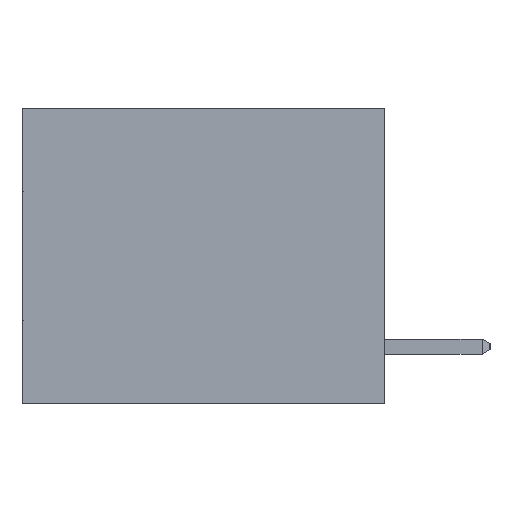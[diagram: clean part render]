
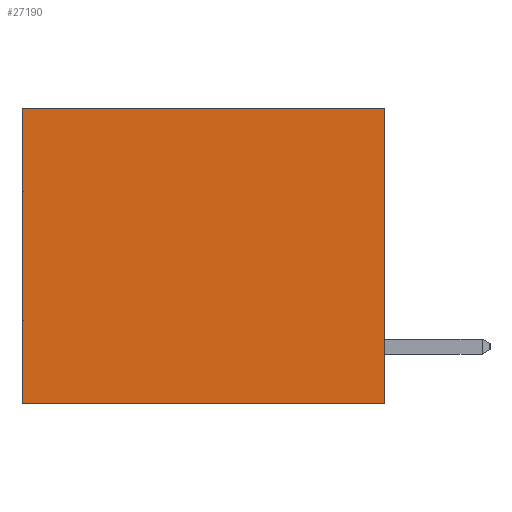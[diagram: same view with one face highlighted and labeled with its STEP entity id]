
A CAD part, left-side view. The second image highlights one B-rep face of the part: STEP entity #27190.
In plain terms, the highlighted planar face has unit normal (-1, 0, 0).
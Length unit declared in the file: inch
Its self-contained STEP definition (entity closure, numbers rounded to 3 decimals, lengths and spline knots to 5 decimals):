
#193 = DIRECTION ( 'NONE',  ( 0., 1., 0. ) ) ;
#298 = CARTESIAN_POINT ( 'NONE',  ( 0.3165, 0., -0.49 ) ) ;
#2090 = EDGE_CURVE ( 'NONE', #5669, #10678, #21121, .T. ) ;
#2999 = CARTESIAN_POINT ( 'NONE',  ( 0.3165, 0.6, -0.49 ) ) ;
#3808 = VECTOR ( 'NONE', #22911, 39.37008 ) ;
#4365 = DIRECTION ( 'NONE',  ( 0., 0., -1. ) ) ;
#4536 = DIRECTION ( 'NONE',  ( 0., 0., -1. ) ) ;
#5238 = ORIENTED_EDGE ( 'NONE', *, *, #6955, .F. ) ;
#5669 = VERTEX_POINT ( 'NONE', #9580 ) ;
#6796 = ORIENTED_EDGE ( 'NONE', *, *, #2090, .T. ) ;
#6955 = EDGE_CURVE ( 'NONE', #12407, #9660, #8573, .T. ) ;
#7861 = CARTESIAN_POINT ( 'NONE',  ( 0.3165, 0., 0. ) ) ;
#8573 = LINE ( 'NONE', #22320, #17529 ) ;
#9580 = CARTESIAN_POINT ( 'NONE',  ( 0.3165, 0.6, 0. ) ) ;
#9660 = VERTEX_POINT ( 'NONE', #25773 ) ;
#10678 = VERTEX_POINT ( 'NONE', #2999 ) ;
#11215 = DIRECTION ( 'NONE',  ( 1., 0., 0. ) ) ;
#11320 = DIRECTION ( 'NONE',  ( 0., 0., -1. ) ) ;
#11658 = VECTOR ( 'NONE', #193, 39.37008 ) ;
#12407 = VERTEX_POINT ( 'NONE', #7861 ) ;
#13776 = ORIENTED_EDGE ( 'NONE', *, *, #20718, .T. ) ;
#14466 = VECTOR ( 'NONE', #4365, 39.37008 ) ;
#14796 = EDGE_LOOP ( 'NONE', ( #6796, #14963, #5238, #13776 ) ) ;
#14963 = ORIENTED_EDGE ( 'NONE', *, *, #16029, .F. ) ;
#15347 = PLANE ( 'NONE',  #19902 ) ;
#16029 = EDGE_CURVE ( 'NONE', #9660, #10678, #27873, .T. ) ;
#16221 = CARTESIAN_POINT ( 'NONE',  ( 0.3165, 0., -0.49 ) ) ;
#17483 = FACE_OUTER_BOUND ( 'NONE', #14796, .T. ) ;
#17529 = VECTOR ( 'NONE', #4536, 39.37008 ) ;
#18332 = LINE ( 'NONE', #20012, #11658 ) ;
#19902 = AXIS2_PLACEMENT_3D ( 'NONE', #16221, #11215, #11320 ) ;
#20012 = CARTESIAN_POINT ( 'NONE',  ( 0.3165, 0., 0. ) ) ;
#20718 = EDGE_CURVE ( 'NONE', #12407, #5669, #18332, .T. ) ;
#21121 = LINE ( 'NONE', #24012, #14466 ) ;
#22320 = CARTESIAN_POINT ( 'NONE',  ( 0.3165, 0., -0.49 ) ) ;
#22911 = DIRECTION ( 'NONE',  ( 0., 1., 0. ) ) ;
#24012 = CARTESIAN_POINT ( 'NONE',  ( 0.3165, 0.6, -0.49 ) ) ;
#25773 = CARTESIAN_POINT ( 'NONE',  ( 0.3165, 0., -0.49 ) ) ;
#27190 = ADVANCED_FACE ( 'NONE', ( #17483 ), #15347, .F. ) ;
#27873 = LINE ( 'NONE', #298, #3808 ) ;
